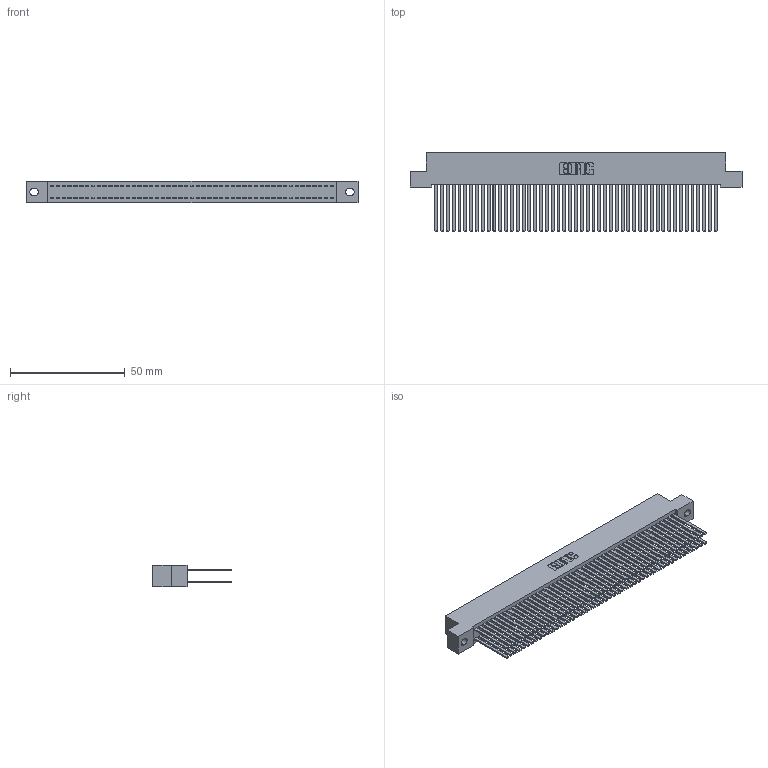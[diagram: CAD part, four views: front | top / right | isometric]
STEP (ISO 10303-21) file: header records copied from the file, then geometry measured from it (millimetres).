
FILE_DESCRIPTION (( 'STEP AP203' ), '1' );
FILE_NAME ('392-098-544-202.STEP', '2018-08-18T11:04:12', ( '' ), ( '' ), 'SwSTEP 2.0', 'SolidWorks 2016', '' );
FILE_SCHEMA (( 'CONFIG_CONTROL_DESIGN' ));
Length unit declared in the file: inch
Products named in the file (3): 342 Part_.128 Slot; 345-292-001_345-293-144; 392-098-544-202
Assembly tree (99 placements, depth 2):
  392-098-544-202
    342 Part_.128 Slot
    345-292-001_345-293-144  x98
Bounding box: 144.78 x 34.3 x 9.4 mm (x, y, z)
Volume: 14363.2 mm3; surface area: 27116.2 mm2
Topology: 99 solids, 99 shells, 4622 faces, 13737 edges, 9026 vertices
Faces by surface type: plane 3206, cylinder 1416
Entity records: 30437 total; most frequent: CARTESIAN_POINT 5034, ORIENTED_EDGE 4970, DIRECTION 4285, EDGE_CURVE 2485, VECTOR 2361, LINE 2361, VERTEX_POINT 1654, AXIS2_PLACEMENT_3D 962
